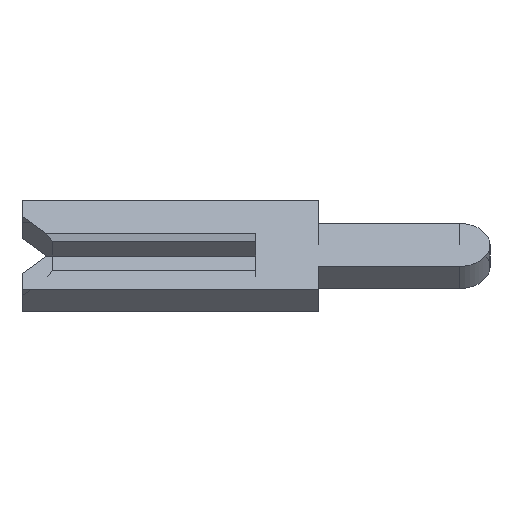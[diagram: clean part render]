
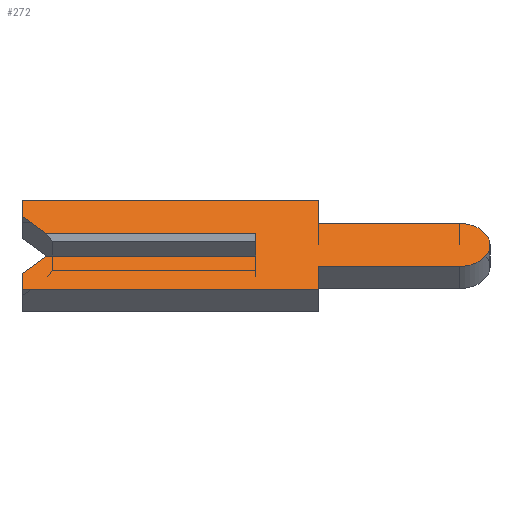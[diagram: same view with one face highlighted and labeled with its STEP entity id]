
A CAD part, left-side view. The second image highlights one B-rep face of the part: STEP entity #272.
In plain terms, the highlighted face is planar.
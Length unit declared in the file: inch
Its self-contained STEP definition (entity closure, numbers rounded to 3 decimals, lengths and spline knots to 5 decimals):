
#9 = CARTESIAN_POINT ( 'NONE',  ( -0.01, 0.15, 0.04 ) ) ;
#21 = CARTESIAN_POINT ( 'NONE',  ( -0.01, 0.134, 0.01 ) ) ;
#29 = VECTOR ( 'NONE', #1705, 39.37008 ) ;
#31 = EDGE_CURVE ( 'NONE', #228, #1299, #1342, .T. ) ;
#50 = VECTOR ( 'NONE', #1722, 39.37008 ) ;
#54 = DIRECTION ( 'NONE',  ( 0., 0., 1. ) ) ;
#58 = DIRECTION ( 'NONE',  ( 1., 0., 0. ) ) ;
#75 = VECTOR ( 'NONE', #1101, 39.37008 ) ;
#90 = PLANE ( 'NONE',  #609 ) ;
#94 = CARTESIAN_POINT ( 'NONE',  ( -0.01, -0.1305, -0.0195 ) ) ;
#99 = EDGE_CURVE ( 'NONE', #583, #1252, #1392, .T. ) ;
#171 = LINE ( 'NONE', #1871, #1641 ) ;
#205 = CARTESIAN_POINT ( 'NONE',  ( -0.01, 0.15, -0.04 ) ) ;
#207 = VERTEX_POINT ( 'NONE', #1720 ) ;
#228 = VERTEX_POINT ( 'NONE', #1732 ) ;
#245 = CARTESIAN_POINT ( 'NONE',  ( -0.01, 0., 0.01 ) ) ;
#271 = VECTOR ( 'NONE', #1430, 39.37008 ) ;
#272 = ADVANCED_FACE ( 'NONE', ( #839 ), #90, .F. ) ;
#277 = EDGE_CURVE ( 'NONE', #558, #228, #676, .T. ) ;
#296 = ORIENTED_EDGE ( 'NONE', *, *, #31, .F. ) ;
#314 = EDGE_CURVE ( 'NONE', #1299, #842, #171, .T. ) ;
#360 = VECTOR ( 'NONE', #1434, 39.37008 ) ;
#365 = ORIENTED_EDGE ( 'NONE', *, *, #1440, .T. ) ;
#376 = CARTESIAN_POINT ( 'NONE',  ( -0.01, 0.15, 0.026 ) ) ;
#390 = DIRECTION ( 'NONE',  ( 0., -1., 0. ) ) ;
#414 = ORIENTED_EDGE ( 'NONE', *, *, #99, .F. ) ;
#432 = ORIENTED_EDGE ( 'NONE', *, *, #572, .F. ) ;
#448 = EDGE_CURVE ( 'NONE', #842, #1280, #744, .T. ) ;
#452 = LINE ( 'NONE', #1317, #50 ) ;
#515 = VERTEX_POINT ( 'NONE', #1680 ) ;
#558 = VERTEX_POINT ( 'NONE', #9 ) ;
#572 = EDGE_CURVE ( 'NONE', #1514, #1366, #1622, .T. ) ;
#583 = VERTEX_POINT ( 'NONE', #21 ) ;
#603 = LINE ( 'NONE', #904, #1173 ) ;
#605 = VERTEX_POINT ( 'NONE', #910 ) ;
#609 = AXIS2_PLACEMENT_3D ( 'NONE', #1149, #58, #1286 ) ;
#612 = CARTESIAN_POINT ( 'NONE',  ( -0.01, 0., 0.0065 ) ) ;
#628 = LINE ( 'NONE', #1591, #931 ) ;
#631 = ORIENTED_EDGE ( 'NONE', *, *, #314, .F. ) ;
#655 = CARTESIAN_POINT ( 'NONE',  ( -0.01, 0.15, 0.026 ) ) ;
#657 = LINE ( 'NONE', #810, #75 ) ;
#673 = CARTESIAN_POINT ( 'NONE',  ( -0.01, 0., -0.01 ) ) ;
#676 = LINE ( 'NONE', #993, #360 ) ;
#717 = EDGE_CURVE ( 'NONE', #1366, #1646, #1482, .T. ) ;
#744 = CIRCLE ( 'NONE', #1699, 0.0195 ) ;
#772 = ORIENTED_EDGE ( 'NONE', *, *, #277, .F. ) ;
#774 = EDGE_CURVE ( 'NONE', #939, #515, #603, .T. ) ;
#782 = CARTESIAN_POINT ( 'NONE',  ( -0.01, -0.1305, -0.01 ) ) ;
#784 = EDGE_CURVE ( 'NONE', #207, #939, #657, .T. ) ;
#786 = CARTESIAN_POINT ( 'NONE',  ( -0.01, -0.04, 0.04 ) ) ;
#810 = CARTESIAN_POINT ( 'NONE',  ( -0.01, 0.15, -0.04 ) ) ;
#839 = FACE_OUTER_BOUND ( 'NONE', #1894, .T. ) ;
#842 = VERTEX_POINT ( 'NONE', #1120 ) ;
#848 = CARTESIAN_POINT ( 'NONE',  ( -0.01, 0.134, -0.01 ) ) ;
#861 = DIRECTION ( 'NONE',  ( 1., 0., 0. ) ) ;
#864 = VECTOR ( 'NONE', #54, 39.37008 ) ;
#890 = ORIENTED_EDGE ( 'NONE', *, *, #448, .F. ) ;
#904 = CARTESIAN_POINT ( 'NONE',  ( -0.01, 0.15, -0.026 ) ) ;
#906 = VECTOR ( 'NONE', #979, 39.37008 ) ;
#910 = CARTESIAN_POINT ( 'NONE',  ( -0.01, -0.04, -0.0195 ) ) ;
#927 = DIRECTION ( 'NONE',  ( 0., -1., 0. ) ) ;
#931 = VECTOR ( 'NONE', #1880, 39.37008 ) ;
#939 = VERTEX_POINT ( 'NONE', #205 ) ;
#962 = CARTESIAN_POINT ( 'NONE',  ( -0.01, 0.1305, 0.0065 ) ) ;
#979 = DIRECTION ( 'NONE',  ( 0., 0., -1. ) ) ;
#983 = ORIENTED_EDGE ( 'NONE', *, *, #1716, .F. ) ;
#993 = CARTESIAN_POINT ( 'NONE',  ( -0.01, 0.15, 0.04 ) ) ;
#1039 = EDGE_CURVE ( 'NONE', #1252, #558, #1248, .T. ) ;
#1056 = ORIENTED_EDGE ( 'NONE', *, *, #784, .F. ) ;
#1061 = DIRECTION ( 'NONE',  ( 0., 0., 1. ) ) ;
#1078 = VECTOR ( 'NONE', #1061, 39.37008 ) ;
#1101 = DIRECTION ( 'NONE',  ( 0., 1., 0. ) ) ;
#1108 = ORIENTED_EDGE ( 'NONE', *, *, #1039, .F. ) ;
#1120 = CARTESIAN_POINT ( 'NONE',  ( -0.01, -0.1305, 0.0195 ) ) ;
#1130 = CARTESIAN_POINT ( 'NONE',  ( -0.01, -0.04, 0.0195 ) ) ;
#1149 = CARTESIAN_POINT ( 'NONE',  ( -0.01, -0.1305, 0. ) ) ;
#1173 = VECTOR ( 'NONE', #1229, 39.37008 ) ;
#1195 = EDGE_CURVE ( 'NONE', #605, #207, #1390, .T. ) ;
#1229 = DIRECTION ( 'NONE',  ( 0., 0., 1. ) ) ;
#1236 = EDGE_CURVE ( 'NONE', #1280, #605, #1533, .T. ) ;
#1248 = LINE ( 'NONE', #655, #864 ) ;
#1252 = VERTEX_POINT ( 'NONE', #376 ) ;
#1274 = ORIENTED_EDGE ( 'NONE', *, *, #1195, .F. ) ;
#1280 = VERTEX_POINT ( 'NONE', #94 ) ;
#1286 = DIRECTION ( 'NONE',  ( 0., 0., -1. ) ) ;
#1299 = VERTEX_POINT ( 'NONE', #1130 ) ;
#1317 = CARTESIAN_POINT ( 'NONE',  ( -0.01, 0.1305, -0.0065 ) ) ;
#1342 = LINE ( 'NONE', #786, #271 ) ;
#1366 = VERTEX_POINT ( 'NONE', #673 ) ;
#1390 = LINE ( 'NONE', #1432, #906 ) ;
#1392 = LINE ( 'NONE', #962, #29 ) ;
#1430 = DIRECTION ( 'NONE',  ( 0., 0., -1. ) ) ;
#1432 = CARTESIAN_POINT ( 'NONE',  ( -0.01, -0.04, -0.04 ) ) ;
#1434 = DIRECTION ( 'NONE',  ( 0., -1., 0. ) ) ;
#1440 = EDGE_CURVE ( 'NONE', #583, #1646, #628, .T. ) ;
#1442 = ORIENTED_EDGE ( 'NONE', *, *, #717, .F. ) ;
#1482 = LINE ( 'NONE', #612, #1078 ) ;
#1514 = VERTEX_POINT ( 'NONE', #848 ) ;
#1533 = LINE ( 'NONE', #1725, #1664 ) ;
#1576 = VECTOR ( 'NONE', #927, 39.37008 ) ;
#1591 = CARTESIAN_POINT ( 'NONE',  ( -0.01, 0.15, 0.01 ) ) ;
#1622 = LINE ( 'NONE', #782, #1576 ) ;
#1641 = VECTOR ( 'NONE', #390, 39.37008 ) ;
#1646 = VERTEX_POINT ( 'NONE', #245 ) ;
#1664 = VECTOR ( 'NONE', #1867, 39.37008 ) ;
#1680 = CARTESIAN_POINT ( 'NONE',  ( -0.01, 0.15, -0.026 ) ) ;
#1699 = AXIS2_PLACEMENT_3D ( 'NONE', #1753, #861, #1903 ) ;
#1705 = DIRECTION ( 'NONE',  ( 0., 0.707, 0.707 ) ) ;
#1716 = EDGE_CURVE ( 'NONE', #515, #1514, #452, .T. ) ;
#1720 = CARTESIAN_POINT ( 'NONE',  ( -0.01, -0.04, -0.04 ) ) ;
#1722 = DIRECTION ( 'NONE',  ( 0., -0.707, 0.707 ) ) ;
#1725 = CARTESIAN_POINT ( 'NONE',  ( -0.01, -0.04, -0.0195 ) ) ;
#1730 = ORIENTED_EDGE ( 'NONE', *, *, #1236, .F. ) ;
#1732 = CARTESIAN_POINT ( 'NONE',  ( -0.01, -0.04, 0.04 ) ) ;
#1753 = CARTESIAN_POINT ( 'NONE',  ( -0.01, -0.1305, 0. ) ) ;
#1821 = ORIENTED_EDGE ( 'NONE', *, *, #774, .F. ) ;
#1867 = DIRECTION ( 'NONE',  ( 0., 1., 0. ) ) ;
#1871 = CARTESIAN_POINT ( 'NONE',  ( -0.01, -0.04, 0.0195 ) ) ;
#1880 = DIRECTION ( 'NONE',  ( 0., -1., 0. ) ) ;
#1894 = EDGE_LOOP ( 'NONE', ( #365, #1442, #432, #983, #1821, #1056, #1274, #1730, #890, #631, #296, #772, #1108, #414 ) ) ;
#1903 = DIRECTION ( 'NONE',  ( 0., 0., -1. ) ) ;
